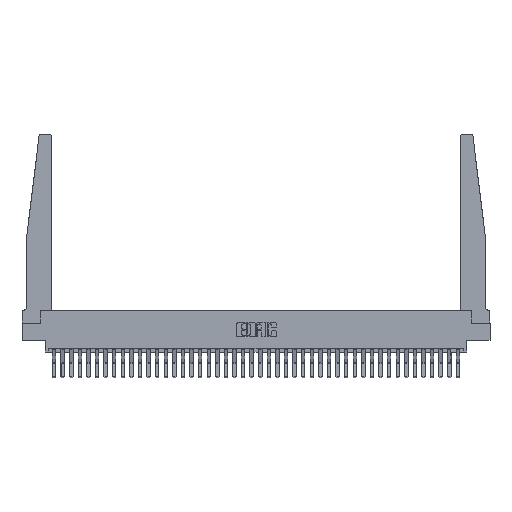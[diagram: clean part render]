
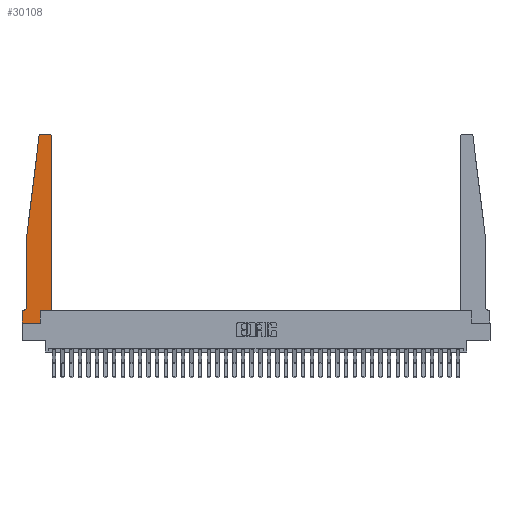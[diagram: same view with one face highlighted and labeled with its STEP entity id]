
A CAD part, top view. The second image highlights one B-rep face of the part: STEP entity #30108.
In plain terms, the highlighted planar face has unit normal (0, 0, 1).
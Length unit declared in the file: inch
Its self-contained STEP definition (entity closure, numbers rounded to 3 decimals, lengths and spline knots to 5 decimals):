
#64 = EDGE_CURVE ( 'NONE', #17236, #13282, #15616, .T. ) ;
#246 = VERTEX_POINT ( 'NONE', #5033 ) ;
#485 = CARTESIAN_POINT ( 'NONE',  ( 0., 0., 0.37 ) ) ;
#1239 = LINE ( 'NONE', #9114, #11767 ) ;
#1413 = DIRECTION ( 'NONE',  ( -1., 0., 0. ) ) ;
#1474 = LINE ( 'NONE', #18450, #10563 ) ;
#2886 = EDGE_CURVE ( 'NONE', #33631, #18145, #13266, .T. ) ;
#3264 = ORIENTED_EDGE ( 'NONE', *, *, #10889, .T. ) ;
#3381 = VECTOR ( 'NONE', #6876, 39.37008 ) ;
#3668 = CARTESIAN_POINT ( 'NONE',  ( 0.395, 2.72, 0.37 ) ) ;
#4322 = EDGE_CURVE ( 'NONE', #13451, #9277, #22340, .T. ) ;
#4489 = CARTESIAN_POINT ( 'NONE',  ( 0., 0., 0.37 ) ) ;
#4828 = ORIENTED_EDGE ( 'NONE', *, *, #17450, .T. ) ;
#5033 = CARTESIAN_POINT ( 'NONE',  ( 0.065, 1.25, 0.37 ) ) ;
#5827 = VECTOR ( 'NONE', #35520, 39.37008 ) ;
#6876 = DIRECTION ( 'NONE',  ( 0., -1., 0. ) ) ;
#8092 = VECTOR ( 'NONE', #30659, 39.37008 ) ;
#8304 = CARTESIAN_POINT ( 'NONE',  ( 0.425, 0.18, 0.37 ) ) ;
#8394 = ORIENTED_EDGE ( 'NONE', *, *, #64, .T. ) ;
#8455 = CARTESIAN_POINT ( 'NONE',  ( 0.425, 0.18, 0.37 ) ) ;
#9011 = EDGE_LOOP ( 'NONE', ( #34937, #29411, #27900, #4828, #19736, #35850, #8394, #9504, #21754, #19130, #29585, #3264 ) ) ;
#9114 = CARTESIAN_POINT ( 'NONE',  ( 0.25, 2.75, 0.37 ) ) ;
#9161 = DIRECTION ( 'NONE',  ( 0., 0., 1. ) ) ;
#9170 = VECTOR ( 'NONE', #35916, 39.37008 ) ;
#9277 = VERTEX_POINT ( 'NONE', #20769 ) ;
#9504 = ORIENTED_EDGE ( 'NONE', *, *, #31725, .T. ) ;
#10563 = VECTOR ( 'NONE', #29530, 39.37008 ) ;
#10889 = EDGE_CURVE ( 'NONE', #9277, #29372, #23983, .T. ) ;
#11236 = PLANE ( 'NONE',  #16389 ) ;
#11353 = LINE ( 'NONE', #8455, #8092 ) ;
#11767 = VECTOR ( 'NONE', #1413, 39.37008 ) ;
#12086 = EDGE_CURVE ( 'NONE', #18145, #246, #26302, .T. ) ;
#12440 = CARTESIAN_POINT ( 'NONE',  ( 0.27653, 2.75, 0.37 ) ) ;
#13209 = DIRECTION ( 'NONE',  ( 0., 0., 1. ) ) ;
#13266 = CIRCLE ( 'NONE', #34186, 0.03 ) ;
#13282 = VERTEX_POINT ( 'NONE', #485 ) ;
#13428 = FACE_OUTER_BOUND ( 'NONE', #9011, .T. ) ;
#13451 = VERTEX_POINT ( 'NONE', #31647 ) ;
#14926 = VERTEX_POINT ( 'NONE', #25939 ) ;
#15616 = LINE ( 'NONE', #4489, #3381 ) ;
#16272 = VERTEX_POINT ( 'NONE', #21489 ) ;
#16364 = LINE ( 'NONE', #24755, #26811 ) ;
#16389 = AXIS2_PLACEMENT_3D ( 'NONE', #22545, #24904, #25264 ) ;
#16532 = VECTOR ( 'NONE', #23940, 39.37008 ) ;
#16962 = DIRECTION ( 'NONE',  ( 0., 0., -1. ) ) ;
#17004 = AXIS2_PLACEMENT_3D ( 'NONE', #3668, #9161, #22645 ) ;
#17236 = VERTEX_POINT ( 'NONE', #32687 ) ;
#17450 = EDGE_CURVE ( 'NONE', #246, #14926, #19757, .T. ) ;
#18145 = VERTEX_POINT ( 'NONE', #21278 ) ;
#18450 = CARTESIAN_POINT ( 'NONE',  ( 0., 0., 0.37 ) ) ;
#18453 = LINE ( 'NONE', #29367, #5827 ) ;
#19108 = VECTOR ( 'NONE', #33421, 39.37008 ) ;
#19130 = ORIENTED_EDGE ( 'NONE', *, *, #20556, .T. ) ;
#19562 = EDGE_CURVE ( 'NONE', #34154, #17236, #16364, .T. ) ;
#19736 = ORIENTED_EDGE ( 'NONE', *, *, #28154, .T. ) ;
#19757 = LINE ( 'NONE', #25384, #9170 ) ;
#19905 = CARTESIAN_POINT ( 'NONE',  ( 0.395, 2.75, 0.37 ) ) ;
#20556 = EDGE_CURVE ( 'NONE', #16272, #13451, #11353, .T. ) ;
#20769 = CARTESIAN_POINT ( 'NONE',  ( 0.425, 2.72, 0.37 ) ) ;
#20966 = CIRCLE ( 'NONE', #27947, 0.05 ) ;
#21278 = CARTESIAN_POINT ( 'NONE',  ( 0.24675, 2.72367, 0.37 ) ) ;
#21489 = CARTESIAN_POINT ( 'NONE',  ( 0.2605, 0.18, 0.37 ) ) ;
#21754 = ORIENTED_EDGE ( 'NONE', *, *, #28111, .T. ) ;
#22340 = LINE ( 'NONE', #8304, #19108 ) ;
#22545 = CARTESIAN_POINT ( 'NONE',  ( 0., 0.1875, 0.37 ) ) ;
#22645 = DIRECTION ( 'NONE',  ( 1., 0., 0. ) ) ;
#23582 = CARTESIAN_POINT ( 'NONE',  ( 0.065, 1.25, 0.37 ) ) ;
#23619 = CARTESIAN_POINT ( 'NONE',  ( 0.27653, 2.72, 0.37 ) ) ;
#23940 = DIRECTION ( 'NONE',  ( -0.122, -0.992, 0. ) ) ;
#23983 = CIRCLE ( 'NONE', #17004, 0.03 ) ;
#24755 = CARTESIAN_POINT ( 'NONE',  ( 0.065, 0.1875, 0.37 ) ) ;
#24904 = DIRECTION ( 'NONE',  ( 0., 0., 1. ) ) ;
#25162 = CARTESIAN_POINT ( 'NONE',  ( 0.015, 0.2375, 0.37 ) ) ;
#25264 = DIRECTION ( 'NONE',  ( 1., 0., 0. ) ) ;
#25384 = CARTESIAN_POINT ( 'NONE',  ( 0.065, 1.25, 0.37 ) ) ;
#25939 = CARTESIAN_POINT ( 'NONE',  ( 0.065, 0.2375, 0.37 ) ) ;
#26302 = LINE ( 'NONE', #23582, #16532 ) ;
#26811 = VECTOR ( 'NONE', #35829, 39.37008 ) ;
#27900 = ORIENTED_EDGE ( 'NONE', *, *, #12086, .T. ) ;
#27947 = AXIS2_PLACEMENT_3D ( 'NONE', #25162, #16962, #35873 ) ;
#28111 = EDGE_CURVE ( 'NONE', #35314, #16272, #18453, .T. ) ;
#28154 = EDGE_CURVE ( 'NONE', #14926, #34154, #20966, .T. ) ;
#29367 = CARTESIAN_POINT ( 'NONE',  ( 0.2605, 0.18, 0.37 ) ) ;
#29372 = VERTEX_POINT ( 'NONE', #19905 ) ;
#29411 = ORIENTED_EDGE ( 'NONE', *, *, #2886, .T. ) ;
#29530 = DIRECTION ( 'NONE',  ( 1., 0., 0. ) ) ;
#29585 = ORIENTED_EDGE ( 'NONE', *, *, #4322, .T. ) ;
#30108 = ADVANCED_FACE ( 'NONE', ( #13428 ), #11236, .T. ) ;
#30659 = DIRECTION ( 'NONE',  ( 1., 0., 0. ) ) ;
#31071 = EDGE_CURVE ( 'NONE', #29372, #33631, #1239, .T. ) ;
#31647 = CARTESIAN_POINT ( 'NONE',  ( 0.425, 0.18, 0.37 ) ) ;
#31725 = EDGE_CURVE ( 'NONE', #13282, #35314, #1474, .T. ) ;
#32687 = CARTESIAN_POINT ( 'NONE',  ( 0., 0.1875, 0.37 ) ) ;
#33421 = DIRECTION ( 'NONE',  ( 0., 1., 0. ) ) ;
#33631 = VERTEX_POINT ( 'NONE', #12440 ) ;
#34154 = VERTEX_POINT ( 'NONE', #34911 ) ;
#34186 = AXIS2_PLACEMENT_3D ( 'NONE', #23619, #13209, #35222 ) ;
#34444 = CARTESIAN_POINT ( 'NONE',  ( 0.2605, 0., 0.37 ) ) ;
#34911 = CARTESIAN_POINT ( 'NONE',  ( 0.015, 0.1875, 0.37 ) ) ;
#34937 = ORIENTED_EDGE ( 'NONE', *, *, #31071, .T. ) ;
#35222 = DIRECTION ( 'NONE',  ( 1., 0., 0. ) ) ;
#35314 = VERTEX_POINT ( 'NONE', #34444 ) ;
#35520 = DIRECTION ( 'NONE',  ( 0., 1., 0. ) ) ;
#35829 = DIRECTION ( 'NONE',  ( -1., 0., 0. ) ) ;
#35850 = ORIENTED_EDGE ( 'NONE', *, *, #19562, .T. ) ;
#35873 = DIRECTION ( 'NONE',  ( -1., 0., 0. ) ) ;
#35916 = DIRECTION ( 'NONE',  ( 0., -1., 0. ) ) ;
